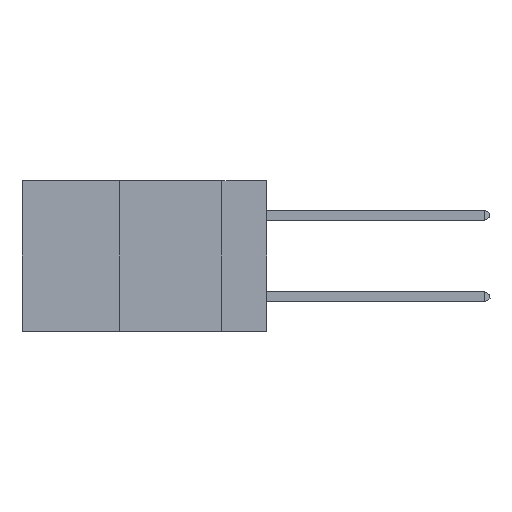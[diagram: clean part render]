
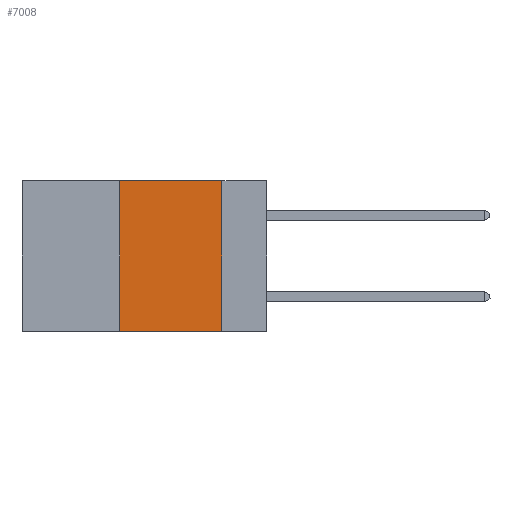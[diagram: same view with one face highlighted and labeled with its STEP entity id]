
A CAD part, left-side view. The second image highlights one B-rep face of the part: STEP entity #7008.
In plain terms, the highlighted planar face has unit normal (-1, 0, 0).
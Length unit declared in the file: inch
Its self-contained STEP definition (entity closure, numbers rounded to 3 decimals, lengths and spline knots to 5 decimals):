
#265 = CARTESIAN_POINT ( 'NONE',  ( 0., 0.6, -0.37 ) ) ;
#975 = EDGE_CURVE ( 'NONE', #3334, #8918, #8138, .T. ) ;
#1549 = CARTESIAN_POINT ( 'NONE',  ( 0., 0.36, 0. ) ) ;
#1771 = CARTESIAN_POINT ( 'NONE',  ( 0., 0.11, -0.37 ) ) ;
#1968 = CARTESIAN_POINT ( 'NONE',  ( 0., 0.36, 0. ) ) ;
#2123 = VERTEX_POINT ( 'NONE', #1968 ) ;
#2455 = EDGE_CURVE ( 'NONE', #2123, #3334, #6078, .T. ) ;
#2656 = VECTOR ( 'NONE', #3371, 39.37008 ) ;
#3142 = ORIENTED_EDGE ( 'NONE', *, *, #8205, .T. ) ;
#3148 = LINE ( 'NONE', #265, #2656 ) ;
#3270 = DIRECTION ( 'NONE',  ( 0., 0., -1. ) ) ;
#3334 = VERTEX_POINT ( 'NONE', #6891 ) ;
#3371 = DIRECTION ( 'NONE',  ( 0., -1., 0. ) ) ;
#3709 = EDGE_CURVE ( 'NONE', #5780, #2123, #6236, .T. ) ;
#4109 = FACE_OUTER_BOUND ( 'NONE', #6139, .T. ) ;
#4622 = ORIENTED_EDGE ( 'NONE', *, *, #2455, .F. ) ;
#5335 = CARTESIAN_POINT ( 'NONE',  ( 0., 0.11, 0. ) ) ;
#5780 = VERTEX_POINT ( 'NONE', #9854 ) ;
#5884 = ORIENTED_EDGE ( 'NONE', *, *, #3709, .F. ) ;
#5958 = VECTOR ( 'NONE', #6182, 39.37008 ) ;
#6078 = LINE ( 'NONE', #6487, #7497 ) ;
#6139 = EDGE_LOOP ( 'NONE', ( #9004, #4622, #5884, #3142 ) ) ;
#6182 = DIRECTION ( 'NONE',  ( 0., 0., -1. ) ) ;
#6236 = LINE ( 'NONE', #1549, #7366 ) ;
#6327 = DIRECTION ( 'NONE',  ( 0., 0., 1. ) ) ;
#6487 = CARTESIAN_POINT ( 'NONE',  ( 0., 0.6, 0. ) ) ;
#6891 = CARTESIAN_POINT ( 'NONE',  ( 0., 0.11, 0. ) ) ;
#7008 = ADVANCED_FACE ( 'NONE', ( #4109 ), #8111, .F. ) ;
#7366 = VECTOR ( 'NONE', #6327, 39.37008 ) ;
#7497 = VECTOR ( 'NONE', #9614, 39.37008 ) ;
#7870 = AXIS2_PLACEMENT_3D ( 'NONE', #8951, #8038, #3270 ) ;
#8038 = DIRECTION ( 'NONE',  ( 1., 0., 0. ) ) ;
#8111 = PLANE ( 'NONE',  #7870 ) ;
#8138 = LINE ( 'NONE', #5335, #5958 ) ;
#8205 = EDGE_CURVE ( 'NONE', #5780, #8918, #3148, .T. ) ;
#8918 = VERTEX_POINT ( 'NONE', #1771 ) ;
#8951 = CARTESIAN_POINT ( 'NONE',  ( 0., 0.6, 0. ) ) ;
#9004 = ORIENTED_EDGE ( 'NONE', *, *, #975, .F. ) ;
#9614 = DIRECTION ( 'NONE',  ( 0., -1., 0. ) ) ;
#9854 = CARTESIAN_POINT ( 'NONE',  ( 0., 0.36, -0.37 ) ) ;
